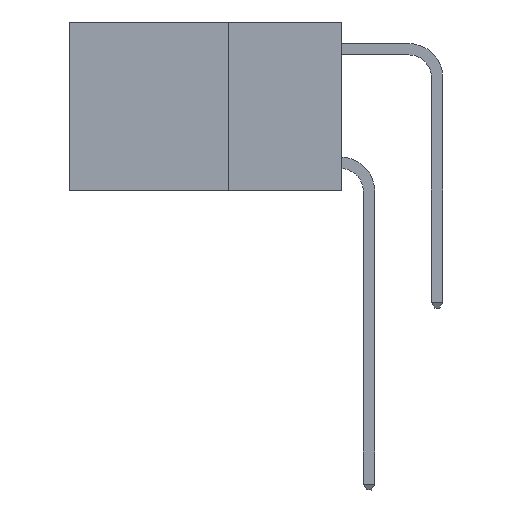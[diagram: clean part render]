
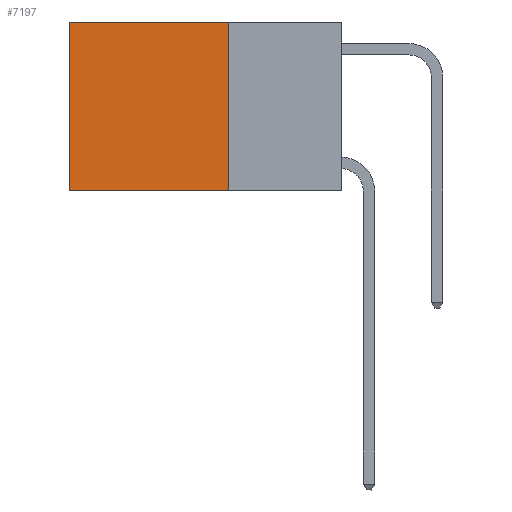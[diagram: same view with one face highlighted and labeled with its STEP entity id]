
A CAD part, left-side view. The second image highlights one B-rep face of the part: STEP entity #7197.
In plain terms, the highlighted planar face has unit normal (-1, 0, 0).
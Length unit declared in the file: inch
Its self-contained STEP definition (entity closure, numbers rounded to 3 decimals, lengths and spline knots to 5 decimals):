
#43 = VERTEX_POINT ( 'NONE', #4313 ) ;
#364 = CARTESIAN_POINT ( 'NONE',  ( 0.2625, 0.6, -0.37 ) ) ;
#449 = VERTEX_POINT ( 'NONE', #11725 ) ;
#517 = AXIS2_PLACEMENT_3D ( 'NONE', #700, #1528, #1652 ) ;
#677 = ORIENTED_EDGE ( 'NONE', *, *, #7452, .T. ) ;
#700 = CARTESIAN_POINT ( 'NONE',  ( 0.2625, 0.25, 0. ) ) ;
#744 = DIRECTION ( 'NONE',  ( 0., 1., 0. ) ) ;
#786 = FACE_OUTER_BOUND ( 'NONE', #5258, .T. ) ;
#1050 = ORIENTED_EDGE ( 'NONE', *, *, #3978, .T. ) ;
#1409 = VECTOR ( 'NONE', #744, 39.37008 ) ;
#1423 = LINE ( 'NONE', #8532, #2536 ) ;
#1528 = DIRECTION ( 'NONE',  ( 1., 0., 0. ) ) ;
#1652 = DIRECTION ( 'NONE',  ( 0., 0., -1. ) ) ;
#2536 = VECTOR ( 'NONE', #12546, 39.37008 ) ;
#2911 = LINE ( 'NONE', #9837, #1409 ) ;
#3884 = LINE ( 'NONE', #5061, #8346 ) ;
#3978 = EDGE_CURVE ( 'NONE', #8806, #4346, #1423, .T. ) ;
#4313 = CARTESIAN_POINT ( 'NONE',  ( 0.2625, 0.25, 0. ) ) ;
#4346 = VERTEX_POINT ( 'NONE', #364 ) ;
#5061 = CARTESIAN_POINT ( 'NONE',  ( 0.2625, 0.25, 0. ) ) ;
#5258 = EDGE_LOOP ( 'NONE', ( #1050, #5555, #12519, #677 ) ) ;
#5555 = ORIENTED_EDGE ( 'NONE', *, *, #11046, .F. ) ;
#6336 = LINE ( 'NONE', #6398, #12388 ) ;
#6398 = CARTESIAN_POINT ( 'NONE',  ( 0.2625, 0.25, 0. ) ) ;
#6664 = PLANE ( 'NONE',  #517 ) ;
#7197 = ADVANCED_FACE ( 'NONE', ( #786 ), #6664, .F. ) ;
#7452 = EDGE_CURVE ( 'NONE', #43, #8806, #3884, .T. ) ;
#8346 = VECTOR ( 'NONE', #11879, 39.37008 ) ;
#8532 = CARTESIAN_POINT ( 'NONE',  ( 0.2625, 0.6, 0. ) ) ;
#8806 = VERTEX_POINT ( 'NONE', #9129 ) ;
#9129 = CARTESIAN_POINT ( 'NONE',  ( 0.2625, 0.6, 0. ) ) ;
#9837 = CARTESIAN_POINT ( 'NONE',  ( 0.2625, 0.25, -0.37 ) ) ;
#9895 = EDGE_CURVE ( 'NONE', #43, #449, #6336, .T. ) ;
#10433 = DIRECTION ( 'NONE',  ( 0., 0., -1. ) ) ;
#11046 = EDGE_CURVE ( 'NONE', #449, #4346, #2911, .T. ) ;
#11725 = CARTESIAN_POINT ( 'NONE',  ( 0.2625, 0.25, -0.37 ) ) ;
#11879 = DIRECTION ( 'NONE',  ( 0., 1., 0. ) ) ;
#12388 = VECTOR ( 'NONE', #10433, 39.37008 ) ;
#12519 = ORIENTED_EDGE ( 'NONE', *, *, #9895, .F. ) ;
#12546 = DIRECTION ( 'NONE',  ( 0., 0., -1. ) ) ;
